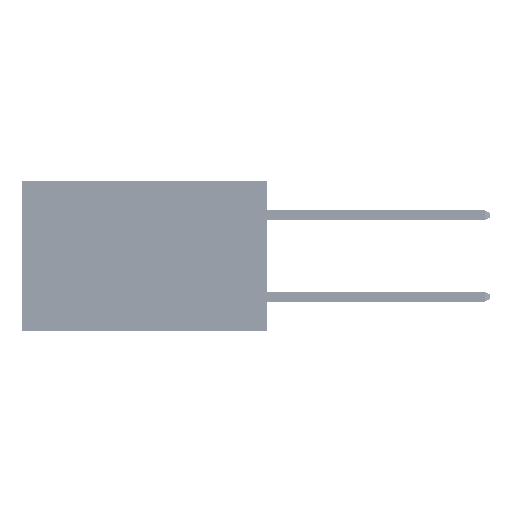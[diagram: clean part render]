
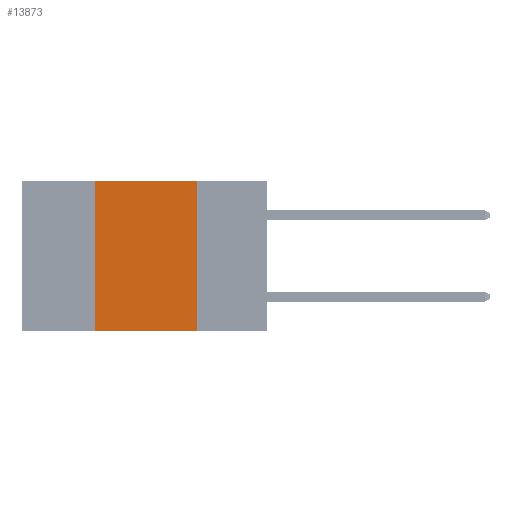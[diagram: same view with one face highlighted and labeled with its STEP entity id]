
A CAD part, left-side view. The second image highlights one B-rep face of the part: STEP entity #13873.
In plain terms, the highlighted planar face has unit normal (-1, 0, 0).
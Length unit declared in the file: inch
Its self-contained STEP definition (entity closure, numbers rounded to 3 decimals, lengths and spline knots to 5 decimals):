
#47 = LINE ( 'NONE', #26624, #637 ) ;
#637 = VECTOR ( 'NONE', #42197, 39.37008 ) ;
#937 = PLANE ( 'NONE',  #47688 ) ;
#1295 = VECTOR ( 'NONE', #32009, 39.37008 ) ;
#2414 = CARTESIAN_POINT ( 'NONE',  ( 0., 0.17, 0. ) ) ;
#3997 = FACE_OUTER_BOUND ( 'NONE', #49459, .T. ) ;
#4324 = CARTESIAN_POINT ( 'NONE',  ( 0., 0.6, -0.37 ) ) ;
#4385 = DIRECTION ( 'NONE',  ( 0., 0., -1. ) ) ;
#4894 = CARTESIAN_POINT ( 'NONE',  ( 0., 0.6, 0. ) ) ;
#4903 = ORIENTED_EDGE ( 'NONE', *, *, #26874, .T. ) ;
#9455 = VERTEX_POINT ( 'NONE', #40959 ) ;
#12655 = VERTEX_POINT ( 'NONE', #48350 ) ;
#13873 = ADVANCED_FACE ( 'NONE', ( #3997 ), #937, .F. ) ;
#17077 = LINE ( 'NONE', #2414, #36884 ) ;
#18384 = EDGE_CURVE ( 'NONE', #9455, #23964, #30859, .T. ) ;
#23964 = VERTEX_POINT ( 'NONE', #25113 ) ;
#25113 = CARTESIAN_POINT ( 'NONE',  ( 0., 0.17, 0. ) ) ;
#25123 = CARTESIAN_POINT ( 'NONE',  ( 0., 0.42, -0.37 ) ) ;
#25186 = VERTEX_POINT ( 'NONE', #25123 ) ;
#26525 = VECTOR ( 'NONE', #43058, 39.37008 ) ;
#26624 = CARTESIAN_POINT ( 'NONE',  ( 0., 0.42, 0. ) ) ;
#26874 = EDGE_CURVE ( 'NONE', #25186, #12655, #47155, .T. ) ;
#28332 = EDGE_CURVE ( 'NONE', #23964, #12655, #17077, .T. ) ;
#30859 = LINE ( 'NONE', #50909, #26525 ) ;
#31784 = EDGE_CURVE ( 'NONE', #25186, #9455, #47, .T. ) ;
#32009 = DIRECTION ( 'NONE',  ( 0., -1., 0. ) ) ;
#36057 = DIRECTION ( 'NONE',  ( 1., 0., 0. ) ) ;
#36094 = ORIENTED_EDGE ( 'NONE', *, *, #18384, .F. ) ;
#36884 = VECTOR ( 'NONE', #50053, 39.37008 ) ;
#40310 = ORIENTED_EDGE ( 'NONE', *, *, #31784, .F. ) ;
#40959 = CARTESIAN_POINT ( 'NONE',  ( 0., 0.42, 0. ) ) ;
#41508 = ORIENTED_EDGE ( 'NONE', *, *, #28332, .F. ) ;
#42197 = DIRECTION ( 'NONE',  ( 0., 0., 1. ) ) ;
#43058 = DIRECTION ( 'NONE',  ( 0., -1., 0. ) ) ;
#47155 = LINE ( 'NONE', #4324, #1295 ) ;
#47688 = AXIS2_PLACEMENT_3D ( 'NONE', #4894, #36057, #4385 ) ;
#48350 = CARTESIAN_POINT ( 'NONE',  ( 0., 0.17, -0.37 ) ) ;
#49459 = EDGE_LOOP ( 'NONE', ( #41508, #36094, #40310, #4903 ) ) ;
#50053 = DIRECTION ( 'NONE',  ( 0., 0., -1. ) ) ;
#50909 = CARTESIAN_POINT ( 'NONE',  ( 0., 0.6, 0. ) ) ;
